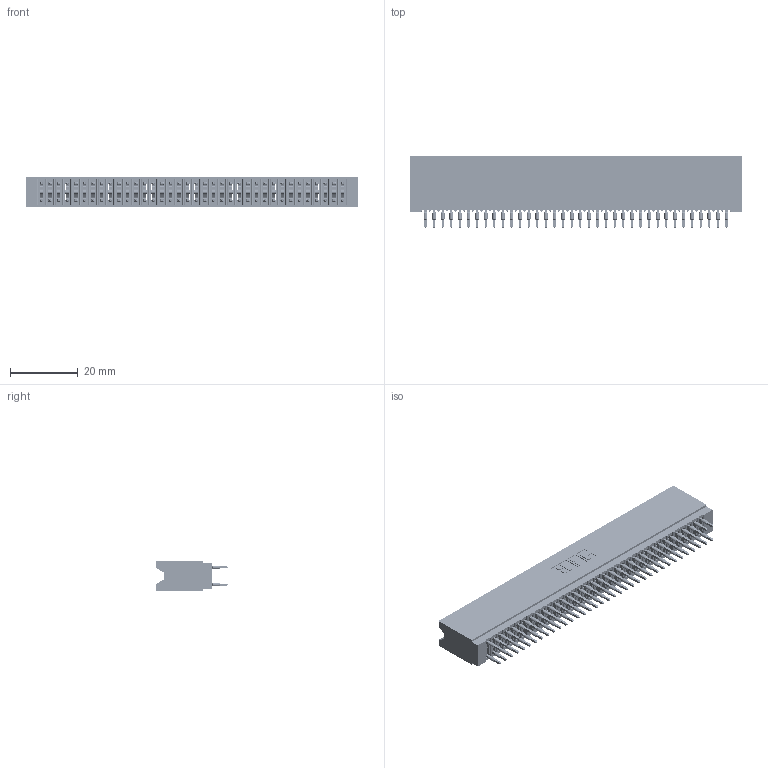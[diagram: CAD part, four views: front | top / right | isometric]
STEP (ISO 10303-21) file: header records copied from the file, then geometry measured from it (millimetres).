
FILE_DESCRIPTION (( 'STEP AP203' ), '1' );
FILE_NAME ('745-072-560-206.STEP', '2026-02-26T19:59:26', ( '' ), ( '' ), 'SwSTEP 2.0', 'SolidWorks 2023', '' );
FILE_SCHEMA (( 'CONFIG_CONTROL_DESIGN' ));
Length unit declared in the file: millimetre
Products named in the file (3): 745-072-560-206; 745 Part_Insulator Option - 06; 745-292-001_560
Assembly tree (73 placements, depth 2):
  745-072-560-206
    745 Part_Insulator Option - 06
    745-292-001_560  x72
Bounding box: 98.04 x 21.22 x 8.89 mm (x, y, z)
Volume: 9109.6 mm3; surface area: 19543.3 mm2
Topology: 73 solids, 73 shells, 7188 faces, 19664 edges, 12484 vertices
Faces by surface type: plane 3728, cylinder 1588, bspline 1440, torus 432
Entity records: 61769 total; most frequent: CARTESIAN_POINT 11220, ORIENTED_EDGE 10644, DIRECTION 9308, EDGE_CURVE 5322, LINE 4916, VECTOR 4916, VERTEX_POINT 3396, AXIS2_PLACEMENT_3D 2196
